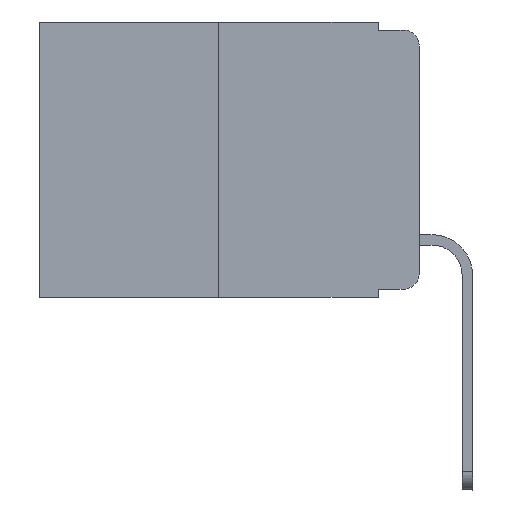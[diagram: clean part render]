
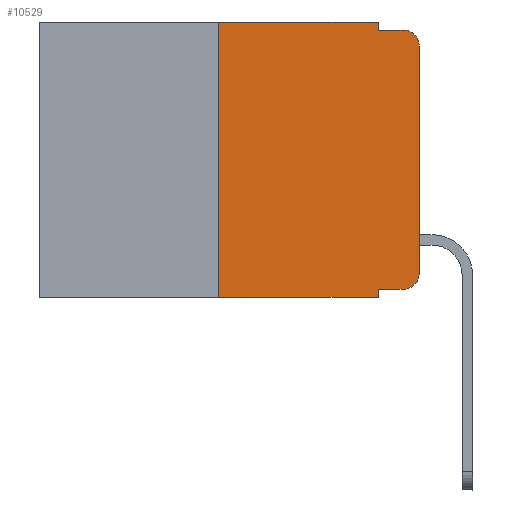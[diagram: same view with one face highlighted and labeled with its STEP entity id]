
A CAD part, left-side view. The second image highlights one B-rep face of the part: STEP entity #10529.
In plain terms, the highlighted planar face has unit normal (-1, 0, 0).
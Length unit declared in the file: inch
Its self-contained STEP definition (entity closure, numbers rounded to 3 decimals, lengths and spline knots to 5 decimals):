
#120 = EDGE_CURVE ( 'NONE', #5472, #7530, #4867, .T. ) ;
#399 = CARTESIAN_POINT ( 'NONE',  ( 0., 0.02, -0.333 ) ) ;
#421 = VECTOR ( 'NONE', #774, 39.37008 ) ;
#440 = CARTESIAN_POINT ( 'NONE',  ( 0., 0.051, -0.01 ) ) ;
#479 = CARTESIAN_POINT ( 'NONE',  ( 0., 0.051, -0.343 ) ) ;
#568 = ORIENTED_EDGE ( 'NONE', *, *, #15076, .T. ) ;
#618 = CARTESIAN_POINT ( 'NONE',  ( 0., 0.25, 0. ) ) ;
#774 = DIRECTION ( 'NONE',  ( 0., 0., 1. ) ) ;
#987 = CARTESIAN_POINT ( 'NONE',  ( 0., 0.473, 0. ) ) ;
#1047 = VERTEX_POINT ( 'NONE', #2439 ) ;
#1464 = VERTEX_POINT ( 'NONE', #15166 ) ;
#1550 = CARTESIAN_POINT ( 'NONE',  ( 0., 0.051, 0. ) ) ;
#1728 = DIRECTION ( 'NONE',  ( -1., 0., 0. ) ) ;
#2205 = AXIS2_PLACEMENT_3D ( 'NONE', #14390, #3817, #6294 ) ;
#2439 = CARTESIAN_POINT ( 'NONE',  ( 0., 0., -0.03 ) ) ;
#2883 = ORIENTED_EDGE ( 'NONE', *, *, #8798, .T. ) ;
#3121 = EDGE_CURVE ( 'NONE', #6521, #12778, #12296, .T. ) ;
#3206 = EDGE_CURVE ( 'NONE', #3424, #5799, #12374, .T. ) ;
#3238 = LINE ( 'NONE', #987, #14093 ) ;
#3358 = ORIENTED_EDGE ( 'NONE', *, *, #7815, .T. ) ;
#3424 = VERTEX_POINT ( 'NONE', #6263 ) ;
#3518 = DIRECTION ( 'NONE',  ( 0., -1., 0. ) ) ;
#3762 = EDGE_CURVE ( 'NONE', #5799, #6521, #3238, .T. ) ;
#3817 = DIRECTION ( 'NONE',  ( 1., 0., 0. ) ) ;
#4188 = ORIENTED_EDGE ( 'NONE', *, *, #120, .F. ) ;
#4265 = VECTOR ( 'NONE', #9793, 39.37008 ) ;
#4330 = DIRECTION ( 'NONE',  ( 0., -1., 0. ) ) ;
#4350 = DIRECTION ( 'NONE',  ( 0., 0., -1. ) ) ;
#4418 = CARTESIAN_POINT ( 'NONE',  ( 0., 0.051, -0.01 ) ) ;
#4560 = EDGE_CURVE ( 'NONE', #11783, #1464, #9183, .T. ) ;
#4867 = LINE ( 'NONE', #1550, #5262 ) ;
#4964 = FACE_OUTER_BOUND ( 'NONE', #7724, .T. ) ;
#5169 = ORIENTED_EDGE ( 'NONE', *, *, #3206, .F. ) ;
#5262 = VECTOR ( 'NONE', #6192, 39.37008 ) ;
#5375 = ORIENTED_EDGE ( 'NONE', *, *, #13962, .T. ) ;
#5472 = VERTEX_POINT ( 'NONE', #8363 ) ;
#5799 = VERTEX_POINT ( 'NONE', #9772 ) ;
#5867 = VECTOR ( 'NONE', #13147, 39.37008 ) ;
#6192 = DIRECTION ( 'NONE',  ( 0., 0., -1. ) ) ;
#6263 = CARTESIAN_POINT ( 'NONE',  ( 0., 0.25, -0.343 ) ) ;
#6294 = DIRECTION ( 'NONE',  ( 0., 0., -1. ) ) ;
#6329 = LINE ( 'NONE', #10107, #4265 ) ;
#6513 = CARTESIAN_POINT ( 'NONE',  ( 0., 0.051, 0. ) ) ;
#6521 = VERTEX_POINT ( 'NONE', #12986 ) ;
#6527 = CARTESIAN_POINT ( 'NONE',  ( 0., 0.02, -0.01 ) ) ;
#6695 = DIRECTION ( 'NONE',  ( 0., 0., -1. ) ) ;
#7530 = VERTEX_POINT ( 'NONE', #479 ) ;
#7590 = CARTESIAN_POINT ( 'NONE',  ( 0., 0.02, -0.03 ) ) ;
#7661 = VERTEX_POINT ( 'NONE', #6527 ) ;
#7724 = EDGE_LOOP ( 'NONE', ( #568, #2883, #9766, #10745, #15031, #5169, #3358, #4188, #5375, #13137 ) ) ;
#7815 = EDGE_CURVE ( 'NONE', #3424, #7530, #10826, .T. ) ;
#8363 = CARTESIAN_POINT ( 'NONE',  ( 0., 0.051, -0.333 ) ) ;
#8798 = EDGE_CURVE ( 'NONE', #1047, #7661, #10566, .T. ) ;
#8864 = LINE ( 'NONE', #4418, #11374 ) ;
#8894 = CARTESIAN_POINT ( 'NONE',  ( 0., 0.02, -0.313 ) ) ;
#9183 = CIRCLE ( 'NONE', #10431, 0.02 ) ;
#9670 = PLANE ( 'NONE',  #2205 ) ;
#9766 = ORIENTED_EDGE ( 'NONE', *, *, #12264, .F. ) ;
#9772 = CARTESIAN_POINT ( 'NONE',  ( 0., 0.25, 0. ) ) ;
#9793 = DIRECTION ( 'NONE',  ( 0., 0., 1. ) ) ;
#10107 = CARTESIAN_POINT ( 'NONE',  ( 0., 0., 0. ) ) ;
#10160 = DIRECTION ( 'NONE',  ( -1., 0., 0. ) ) ;
#10208 = DIRECTION ( 'NONE',  ( 0., -1., 0. ) ) ;
#10309 = VECTOR ( 'NONE', #4350, 39.37008 ) ;
#10431 = AXIS2_PLACEMENT_3D ( 'NONE', #8894, #10160, #6695 ) ;
#10471 = CARTESIAN_POINT ( 'NONE',  ( 0., 0.051, -0.333 ) ) ;
#10529 = ADVANCED_FACE ( 'NONE', ( #4964 ), #9670, .F. ) ;
#10566 = CIRCLE ( 'NONE', #11322, 0.02 ) ;
#10745 = ORIENTED_EDGE ( 'NONE', *, *, #3121, .F. ) ;
#10826 = LINE ( 'NONE', #14606, #5867 ) ;
#11322 = AXIS2_PLACEMENT_3D ( 'NONE', #7590, #1728, #12246 ) ;
#11374 = VECTOR ( 'NONE', #10208, 39.37008 ) ;
#11783 = VERTEX_POINT ( 'NONE', #399 ) ;
#12246 = DIRECTION ( 'NONE',  ( 0., 0., -1. ) ) ;
#12264 = EDGE_CURVE ( 'NONE', #12778, #7661, #8864, .T. ) ;
#12296 = LINE ( 'NONE', #6513, #10309 ) ;
#12374 = LINE ( 'NONE', #618, #421 ) ;
#12778 = VERTEX_POINT ( 'NONE', #440 ) ;
#12986 = CARTESIAN_POINT ( 'NONE',  ( 0., 0.051, 0. ) ) ;
#13137 = ORIENTED_EDGE ( 'NONE', *, *, #4560, .T. ) ;
#13147 = DIRECTION ( 'NONE',  ( 0., -1., 0. ) ) ;
#13962 = EDGE_CURVE ( 'NONE', #5472, #11783, #14023, .T. ) ;
#14023 = LINE ( 'NONE', #10471, #14611 ) ;
#14093 = VECTOR ( 'NONE', #4330, 39.37008 ) ;
#14390 = CARTESIAN_POINT ( 'NONE',  ( 0., 0.473, 0. ) ) ;
#14606 = CARTESIAN_POINT ( 'NONE',  ( 0., 0.473, -0.343 ) ) ;
#14611 = VECTOR ( 'NONE', #3518, 39.37008 ) ;
#15031 = ORIENTED_EDGE ( 'NONE', *, *, #3762, .F. ) ;
#15076 = EDGE_CURVE ( 'NONE', #1464, #1047, #6329, .T. ) ;
#15166 = CARTESIAN_POINT ( 'NONE',  ( 0., 0., -0.313 ) ) ;
